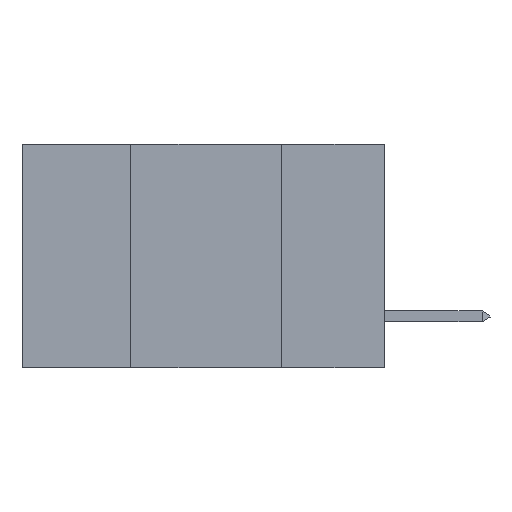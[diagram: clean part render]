
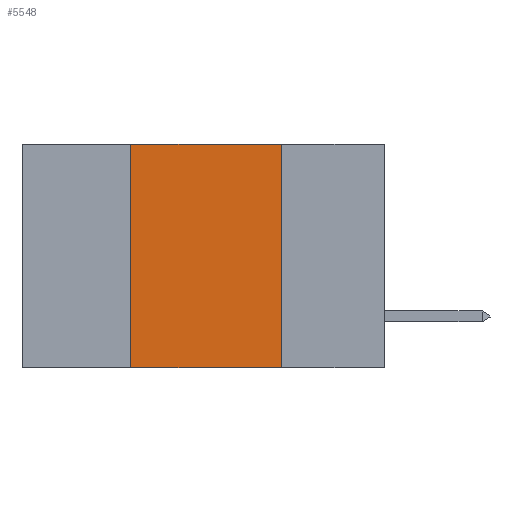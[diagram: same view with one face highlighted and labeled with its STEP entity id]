
A CAD part, left-side view. The second image highlights one B-rep face of the part: STEP entity #5548.
In plain terms, the highlighted planar face has unit normal (-1, 0, 0).
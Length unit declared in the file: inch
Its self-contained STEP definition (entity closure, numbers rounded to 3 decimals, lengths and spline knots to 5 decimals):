
#1359 = CARTESIAN_POINT ( 'NONE',  ( 0., 0.17, 0. ) ) ;
#1874 = DIRECTION ( 'NONE',  ( 0., 0., -1. ) ) ;
#3047 = LINE ( 'NONE', #35917, #13724 ) ;
#5548 = ADVANCED_FACE ( 'NONE', ( #45511 ), #32553, .F. ) ;
#9040 = CARTESIAN_POINT ( 'NONE',  ( 0., 0.17, -0.37 ) ) ;
#9956 = CARTESIAN_POINT ( 'NONE',  ( 0., 0.42, 0. ) ) ;
#12964 = DIRECTION ( 'NONE',  ( 0., 0., -1. ) ) ;
#13724 = VECTOR ( 'NONE', #14577, 39.37008 ) ;
#14577 = DIRECTION ( 'NONE',  ( 0., -1., 0. ) ) ;
#15342 = CARTESIAN_POINT ( 'NONE',  ( 0., 0.6, 0. ) ) ;
#16116 = CARTESIAN_POINT ( 'NONE',  ( 0., 0.17, 0. ) ) ;
#17545 = ORIENTED_EDGE ( 'NONE', *, *, #37368, .T. ) ;
#18385 = CARTESIAN_POINT ( 'NONE',  ( 0., 0.42, 0. ) ) ;
#19580 = ORIENTED_EDGE ( 'NONE', *, *, #46338, .F. ) ;
#19964 = VERTEX_POINT ( 'NONE', #16116 ) ;
#22873 = LINE ( 'NONE', #1359, #45983 ) ;
#24593 = DIRECTION ( 'NONE',  ( 1., 0., 0. ) ) ;
#25260 = VERTEX_POINT ( 'NONE', #18385 ) ;
#25479 = LINE ( 'NONE', #15342, #45109 ) ;
#26554 = DIRECTION ( 'NONE',  ( 0., -1., 0. ) ) ;
#29695 = EDGE_CURVE ( 'NONE', #38956, #25260, #43447, .T. ) ;
#30497 = EDGE_LOOP ( 'NONE', ( #19580, #38589, #39342, #17545 ) ) ;
#32553 = PLANE ( 'NONE',  #41297 ) ;
#34416 = EDGE_CURVE ( 'NONE', #25260, #19964, #25479, .T. ) ;
#34585 = CARTESIAN_POINT ( 'NONE',  ( 0., 0.42, -0.37 ) ) ;
#35917 = CARTESIAN_POINT ( 'NONE',  ( 0., 0.6, -0.37 ) ) ;
#36278 = DIRECTION ( 'NONE',  ( 0., 0., 1. ) ) ;
#36345 = CARTESIAN_POINT ( 'NONE',  ( 0., 0.6, 0. ) ) ;
#37368 = EDGE_CURVE ( 'NONE', #38956, #41299, #3047, .T. ) ;
#38589 = ORIENTED_EDGE ( 'NONE', *, *, #34416, .F. ) ;
#38956 = VERTEX_POINT ( 'NONE', #34585 ) ;
#39342 = ORIENTED_EDGE ( 'NONE', *, *, #29695, .F. ) ;
#41297 = AXIS2_PLACEMENT_3D ( 'NONE', #36345, #24593, #1874 ) ;
#41299 = VERTEX_POINT ( 'NONE', #9040 ) ;
#42889 = VECTOR ( 'NONE', #36278, 39.37008 ) ;
#43447 = LINE ( 'NONE', #9956, #42889 ) ;
#45109 = VECTOR ( 'NONE', #26554, 39.37008 ) ;
#45511 = FACE_OUTER_BOUND ( 'NONE', #30497, .T. ) ;
#45983 = VECTOR ( 'NONE', #12964, 39.37008 ) ;
#46338 = EDGE_CURVE ( 'NONE', #19964, #41299, #22873, .T. ) ;
